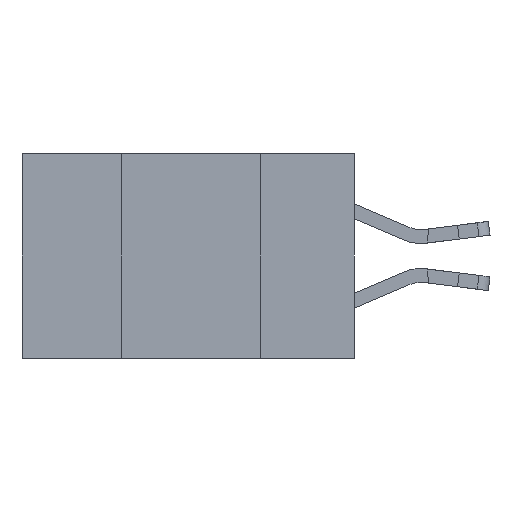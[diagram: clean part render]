
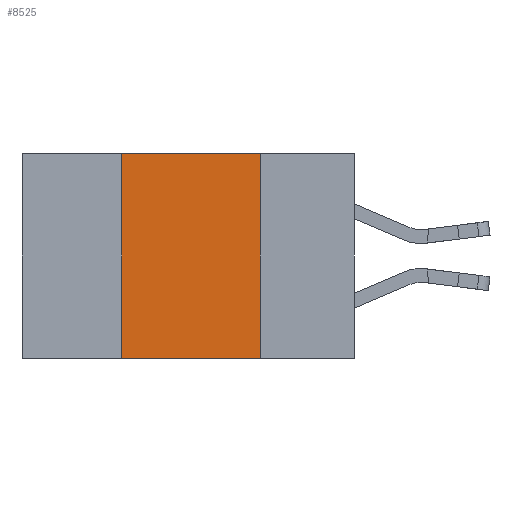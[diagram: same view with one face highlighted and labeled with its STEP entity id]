
A CAD part, left-side view. The second image highlights one B-rep face of the part: STEP entity #8525.
In plain terms, the highlighted planar face has unit normal (-1, 0, 0).
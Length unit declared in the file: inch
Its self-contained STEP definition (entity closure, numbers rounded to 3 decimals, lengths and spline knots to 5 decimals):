
#519 = CARTESIAN_POINT ( 'NONE',  ( 0., 0.6, 0. ) ) ;
#593 = DIRECTION ( 'NONE',  ( 0., -1., 0. ) ) ;
#950 = EDGE_CURVE ( 'NONE', #6163, #21181, #1370, .T. ) ;
#1370 = LINE ( 'NONE', #7316, #10904 ) ;
#1374 = DIRECTION ( 'NONE',  ( 1., 0., 0. ) ) ;
#1513 = LINE ( 'NONE', #519, #9998 ) ;
#3276 = AXIS2_PLACEMENT_3D ( 'NONE', #16737, #1374, #9680 ) ;
#4160 = DIRECTION ( 'NONE',  ( 0., -1., 0. ) ) ;
#4321 = VERTEX_POINT ( 'NONE', #6528 ) ;
#5679 = CARTESIAN_POINT ( 'NONE',  ( 0., 0.17, -0.37 ) ) ;
#6163 = VERTEX_POINT ( 'NONE', #14573 ) ;
#6528 = CARTESIAN_POINT ( 'NONE',  ( 0., 0.17, 0. ) ) ;
#7108 = DIRECTION ( 'NONE',  ( 0., 0., 1. ) ) ;
#7316 = CARTESIAN_POINT ( 'NONE',  ( 0., 0.42, 0. ) ) ;
#7491 = LINE ( 'NONE', #13002, #20031 ) ;
#7615 = EDGE_CURVE ( 'NONE', #4321, #21602, #7491, .T. ) ;
#8100 = LINE ( 'NONE', #12417, #10723 ) ;
#8525 = ADVANCED_FACE ( 'NONE', ( #18126 ), #21653, .F. ) ;
#9680 = DIRECTION ( 'NONE',  ( 0., 0., -1. ) ) ;
#9998 = VECTOR ( 'NONE', #593, 39.37008 ) ;
#10711 = EDGE_CURVE ( 'NONE', #21181, #4321, #1513, .T. ) ;
#10723 = VECTOR ( 'NONE', #4160, 39.37008 ) ;
#10904 = VECTOR ( 'NONE', #7108, 39.37008 ) ;
#10998 = CARTESIAN_POINT ( 'NONE',  ( 0., 0.42, 0. ) ) ;
#11906 = ORIENTED_EDGE ( 'NONE', *, *, #7615, .F. ) ;
#12417 = CARTESIAN_POINT ( 'NONE',  ( 0., 0.6, -0.37 ) ) ;
#12957 = ORIENTED_EDGE ( 'NONE', *, *, #950, .F. ) ;
#13002 = CARTESIAN_POINT ( 'NONE',  ( 0., 0.17, 0. ) ) ;
#14306 = EDGE_LOOP ( 'NONE', ( #11906, #21401, #12957, #20540 ) ) ;
#14573 = CARTESIAN_POINT ( 'NONE',  ( 0., 0.42, -0.37 ) ) ;
#14741 = DIRECTION ( 'NONE',  ( 0., 0., -1. ) ) ;
#16737 = CARTESIAN_POINT ( 'NONE',  ( 0., 0.6, 0. ) ) ;
#18126 = FACE_OUTER_BOUND ( 'NONE', #14306, .T. ) ;
#20031 = VECTOR ( 'NONE', #14741, 39.37008 ) ;
#20540 = ORIENTED_EDGE ( 'NONE', *, *, #21557, .T. ) ;
#21181 = VERTEX_POINT ( 'NONE', #10998 ) ;
#21401 = ORIENTED_EDGE ( 'NONE', *, *, #10711, .F. ) ;
#21557 = EDGE_CURVE ( 'NONE', #6163, #21602, #8100, .T. ) ;
#21602 = VERTEX_POINT ( 'NONE', #5679 ) ;
#21653 = PLANE ( 'NONE',  #3276 ) ;
